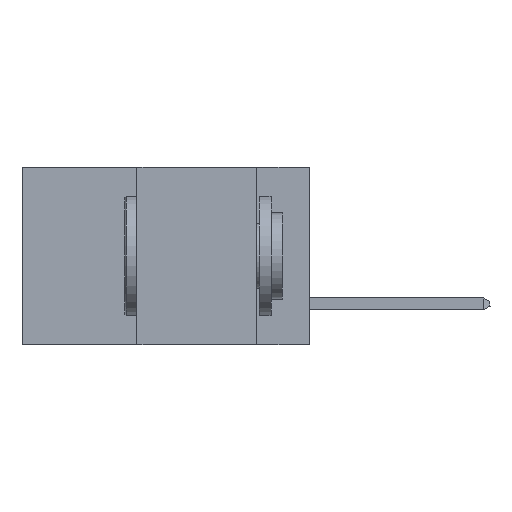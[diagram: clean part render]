
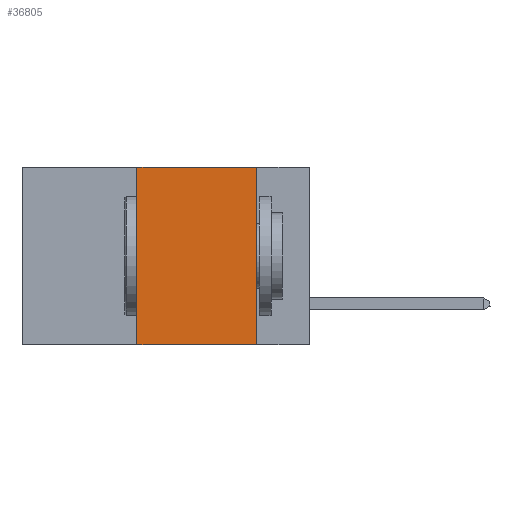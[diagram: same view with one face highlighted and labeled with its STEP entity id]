
A CAD part, left-side view. The second image highlights one B-rep face of the part: STEP entity #36805.
In plain terms, the highlighted planar face has unit normal (-1, 0, 0).
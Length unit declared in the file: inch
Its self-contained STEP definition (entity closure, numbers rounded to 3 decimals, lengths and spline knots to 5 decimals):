
#54 = VERTEX_POINT ( 'NONE', #21776 ) ;
#659 = DIRECTION ( 'NONE',  ( 0., -1., 0. ) ) ;
#2062 = CARTESIAN_POINT ( 'NONE',  ( 0., 0.36, -0.37 ) ) ;
#2948 = DIRECTION ( 'NONE',  ( 1., 0., 0. ) ) ;
#4278 = ORIENTED_EDGE ( 'NONE', *, *, #12687, .F. ) ;
#5748 = VECTOR ( 'NONE', #7398, 39.37008 ) ;
#7398 = DIRECTION ( 'NONE',  ( 0., -1., 0. ) ) ;
#7939 = LINE ( 'NONE', #9034, #15846 ) ;
#8006 = AXIS2_PLACEMENT_3D ( 'NONE', #18372, #2948, #37449 ) ;
#8835 = CARTESIAN_POINT ( 'NONE',  ( 0., 0.11, -0.37 ) ) ;
#8956 = VERTEX_POINT ( 'NONE', #8835 ) ;
#9034 = CARTESIAN_POINT ( 'NONE',  ( 0., 0.36, 0. ) ) ;
#9130 = VERTEX_POINT ( 'NONE', #2062 ) ;
#11543 = CARTESIAN_POINT ( 'NONE',  ( 0., 0.11, 0. ) ) ;
#12149 = PLANE ( 'NONE',  #8006 ) ;
#12687 = EDGE_CURVE ( 'NONE', #9130, #54, #7939, .T. ) ;
#12722 = LINE ( 'NONE', #39369, #5748 ) ;
#15258 = EDGE_CURVE ( 'NONE', #9130, #8956, #12722, .T. ) ;
#15846 = VECTOR ( 'NONE', #19815, 39.37008 ) ;
#16615 = VECTOR ( 'NONE', #659, 39.37008 ) ;
#18372 = CARTESIAN_POINT ( 'NONE',  ( 0., 0.6, 0. ) ) ;
#19055 = ORIENTED_EDGE ( 'NONE', *, *, #15258, .T. ) ;
#19815 = DIRECTION ( 'NONE',  ( 0., 0., 1. ) ) ;
#20963 = DIRECTION ( 'NONE',  ( 0., 0., -1. ) ) ;
#21154 = VERTEX_POINT ( 'NONE', #40341 ) ;
#21776 = CARTESIAN_POINT ( 'NONE',  ( 0., 0.36, 0. ) ) ;
#22479 = CARTESIAN_POINT ( 'NONE',  ( 0., 0.6, 0. ) ) ;
#22541 = LINE ( 'NONE', #22479, #16615 ) ;
#24087 = ORIENTED_EDGE ( 'NONE', *, *, #40001, .F. ) ;
#24935 = EDGE_LOOP ( 'NONE', ( #29762, #24087, #4278, #19055 ) ) ;
#25760 = FACE_OUTER_BOUND ( 'NONE', #24935, .T. ) ;
#29476 = LINE ( 'NONE', #11543, #40900 ) ;
#29762 = ORIENTED_EDGE ( 'NONE', *, *, #34924, .F. ) ;
#34924 = EDGE_CURVE ( 'NONE', #21154, #8956, #29476, .T. ) ;
#36805 = ADVANCED_FACE ( 'NONE', ( #25760 ), #12149, .F. ) ;
#37449 = DIRECTION ( 'NONE',  ( 0., 0., -1. ) ) ;
#39369 = CARTESIAN_POINT ( 'NONE',  ( 0., 0.6, -0.37 ) ) ;
#40001 = EDGE_CURVE ( 'NONE', #54, #21154, #22541, .T. ) ;
#40341 = CARTESIAN_POINT ( 'NONE',  ( 0., 0.11, 0. ) ) ;
#40900 = VECTOR ( 'NONE', #20963, 39.37008 ) ;
